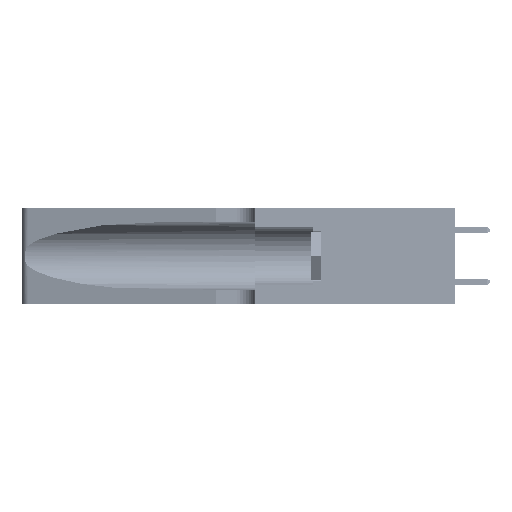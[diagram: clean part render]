
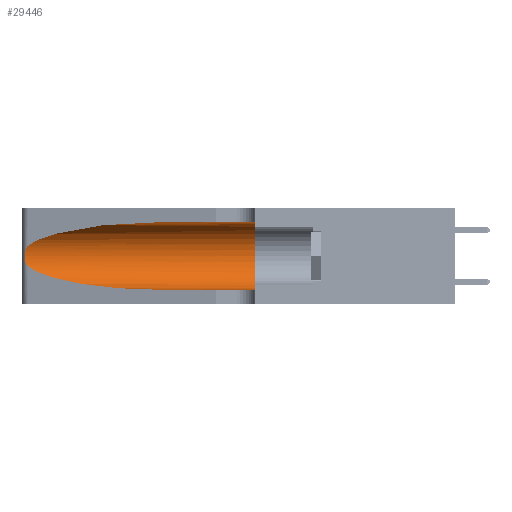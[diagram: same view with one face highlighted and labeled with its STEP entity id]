
A CAD part, left-side view. The second image highlights one B-rep face of the part: STEP entity #29446.
In plain terms, the highlighted cylindrical face has radius 3.308 mm (diameter 6.617 mm), a partial arc.
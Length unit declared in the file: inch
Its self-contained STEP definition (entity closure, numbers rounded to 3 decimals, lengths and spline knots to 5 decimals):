
#840 = ORIENTED_EDGE ( 'NONE', *, *, #49002, .T. ) ;
#1829 = DIRECTION ( 'NONE',  ( 0., 0., -1. ) ) ;
#2271 = EDGE_CURVE ( 'NONE', #34082, #46033, #19145, .T. ) ;
#2732 = LINE ( 'NONE', #43345, #43761 ) ;
#3081 = CARTESIAN_POINT ( 'NONE',  ( 0.25487, 1.22718, 0.22369 ) ) ;
#4306 = CARTESIAN_POINT ( 'NONE',  ( 0.25487, 1.22718, 0.14631 ) ) ;
#5226 = CARTESIAN_POINT ( 'NONE',  ( 0.1305, 0.35, 0.185 ) ) ;
#6212 = CARTESIAN_POINT ( 'NONE',  ( 0.1305, 0.72297, 0.31525 ) ) ;
#6383 = FACE_OUTER_BOUND ( 'NONE', #49997, .T. ) ;
#6954 = LINE ( 'NONE', #20405, #44265 ) ;
#7512 = CARTESIAN_POINT ( 'NONE',  ( 0.25856, 1.23593, 0.16098 ) ) ;
#7681 = CARTESIAN_POINT ( 'NONE',  ( 0.25487, 1.22718, 0.22369 ) ) ;
#7688 = CARTESIAN_POINT ( 'NONE',  ( 0.1305, 0.72297, 0.31525 ) ) ;
#9239 = DIRECTION ( 'NONE',  ( 0., 0., 1. ) ) ;
#9847 = ORIENTED_EDGE ( 'NONE', *, *, #13109, .F. ) ;
#11036 = CARTESIAN_POINT ( 'NONE',  ( 0.25639, 1.23186, 0.15144 ) ) ;
#11256 = ORIENTED_EDGE ( 'NONE', *, *, #45547, .T. ) ;
#13078 = VERTEX_POINT ( 'NONE', #16747 ) ;
#13109 = EDGE_CURVE ( 'NONE', #28854, #35072, #6954, .T. ) ;
#15540 = CARTESIAN_POINT ( 'NONE',  ( 0.25854, 1.2359, 0.20912 ) ) ;
#16747 = CARTESIAN_POINT ( 'NONE',  ( 0.1305, 0.35, 0.05475 ) ) ;
#17426 = CARTESIAN_POINT ( 'NONE',  ( 0.1305, 0.35, 0.31525 ) ) ;
#18692 = CIRCLE ( 'NONE', #24032, 0.13025 ) ;
#19145 = B_SPLINE_CURVE_WITH_KNOTS ( 'NONE', 3,
 ( #7681, #27005, #51390, #31512, #15540, #23680, #43154, #39186, #47032, #7512, #19354, #11036, #23522, #51221 ),
 .UNSPECIFIED., .F., .F.,
 ( 4, 2, 2, 2, 2, 2, 4 ),
 ( 0., 0.00027, 0.00053, 0.00107, 0.0016, 0.00187, 0.00214 ),
 .UNSPECIFIED. ) ;
#19354 = CARTESIAN_POINT ( 'NONE',  ( 0.25789, 1.23486, 0.15765 ) ) ;
#19531 = CARTESIAN_POINT ( 'NONE',  ( 0.2373, 1.15595, 0.28018 ) ) ;
#19809 = CARTESIAN_POINT ( 'NONE',  ( 0.18966, 0.96281, 0.05475 ) ) ;
#20405 = CARTESIAN_POINT ( 'NONE',  ( 0.1305, 1.61858, 0.31525 ) ) ;
#23061 = CARTESIAN_POINT ( 'NONE',  ( 0.25487, 1.22718, 0.14631 ) ) ;
#23522 = CARTESIAN_POINT ( 'NONE',  ( 0.25555, 1.22993, 0.14849 ) ) ;
#23680 = CARTESIAN_POINT ( 'NONE',  ( 0.26018, 1.23835, 0.19895 ) ) ;
#23696 = ORIENTED_EDGE ( 'NONE', *, *, #30982, .T. ) ;
#24032 = AXIS2_PLACEMENT_3D ( 'NONE', #5226, #36570, #9239 ) ;
#25633 = CARTESIAN_POINT ( 'NONE',  ( 0.1305, 1.61858, 0.185 ) ) ;
#27005 = CARTESIAN_POINT ( 'NONE',  ( 0.25555, 1.22994, 0.2215 ) ) ;
#28373 =( BOUNDED_CURVE ( )  B_SPLINE_CURVE ( 3, ( #7688, #47038, #19531, #43333 ),
 .UNSPECIFIED., .F., .F. ) 
 B_SPLINE_CURVE_WITH_KNOTS ( ( 4, 4 ),
 ( 1.5708, 2.84003 ),
 .UNSPECIFIED. ) 
 CURVE ( )  GEOMETRIC_REPRESENTATION_ITEM ( )  RATIONAL_B_SPLINE_CURVE ( ( 1., 0.87, 0.87, 1. ) ) 
 REPRESENTATION_ITEM ( '' )  );
#28854 = VERTEX_POINT ( 'NONE', #6212 ) ;
#29446 = ADVANCED_FACE ( 'NONE', ( #6383 ), #41865, .F. ) ;
#30982 = EDGE_CURVE ( 'NONE', #28854, #34082, #28373, .T. ) ;
#31512 = CARTESIAN_POINT ( 'NONE',  ( 0.25787, 1.23484, 0.2124 ) ) ;
#32303 = CARTESIAN_POINT ( 'NONE',  ( 0.2373, 1.15595, 0.08982 ) ) ;
#33391 = ORIENTED_EDGE ( 'NONE', *, *, #43153, .F. ) ;
#34082 = VERTEX_POINT ( 'NONE', #3081 ) ;
#35072 = VERTEX_POINT ( 'NONE', #17426 ) ;
#36570 = DIRECTION ( 'NONE',  ( 0., 1., 0. ) ) ;
#38183 = CARTESIAN_POINT ( 'NONE',  ( 0.1305, 0.72297, 0.05475 ) ) ;
#39186 = CARTESIAN_POINT ( 'NONE',  ( 0.26075, 1.23896, 0.178 ) ) ;
#39803 = CARTESIAN_POINT ( 'NONE',  ( 0.1305, 0.72297, 0.05475 ) ) ;
#40378 = DIRECTION ( 'NONE',  ( 0., -1., 0. ) ) ;
#41865 = CYLINDRICAL_SURFACE ( 'NONE', #49493, 0.13025 ) ;
#42395 =( BOUNDED_CURVE ( )  B_SPLINE_CURVE ( 3, ( #4306, #32303, #19809, #39803 ),
 .UNSPECIFIED., .F., .T. ) 
 B_SPLINE_CURVE_WITH_KNOTS ( ( 4, 4 ),
 ( 3.44316, 4.71239 ),
 .UNSPECIFIED. ) 
 CURVE ( )  GEOMETRIC_REPRESENTATION_ITEM ( )  RATIONAL_B_SPLINE_CURVE ( ( 1., 0.87, 0.87, 1. ) ) 
 REPRESENTATION_ITEM ( '' )  );
#43153 = EDGE_CURVE ( 'NONE', #35072, #13078, #18692, .T. ) ;
#43154 = CARTESIAN_POINT ( 'NONE',  ( 0.26075, 1.23896, 0.19203 ) ) ;
#43333 = CARTESIAN_POINT ( 'NONE',  ( 0.25487, 1.22718, 0.22369 ) ) ;
#43345 = CARTESIAN_POINT ( 'NONE',  ( 0.1305, 1.61858, 0.05475 ) ) ;
#43507 = DIRECTION ( 'NONE',  ( 0., -1., 0. ) ) ;
#43761 = VECTOR ( 'NONE', #43507, 39.37008 ) ;
#44265 = VECTOR ( 'NONE', #40378, 39.37008 ) ;
#45547 = EDGE_CURVE ( 'NONE', #46033, #46734, #42395, .T. ) ;
#46033 = VERTEX_POINT ( 'NONE', #23061 ) ;
#46734 = VERTEX_POINT ( 'NONE', #38183 ) ;
#47032 = CARTESIAN_POINT ( 'NONE',  ( 0.26017, 1.23833, 0.17102 ) ) ;
#47038 = CARTESIAN_POINT ( 'NONE',  ( 0.18966, 0.96281, 0.31525 ) ) ;
#48053 = ORIENTED_EDGE ( 'NONE', *, *, #2271, .T. ) ;
#49002 = EDGE_CURVE ( 'NONE', #46734, #13078, #2732, .T. ) ;
#49493 = AXIS2_PLACEMENT_3D ( 'NONE', #25633, #50010, #1829 ) ;
#49997 = EDGE_LOOP ( 'NONE', ( #23696, #48053, #11256, #840, #33391, #9847 ) ) ;
#50010 = DIRECTION ( 'NONE',  ( 0., -1., 0. ) ) ;
#51221 = CARTESIAN_POINT ( 'NONE',  ( 0.25487, 1.22718, 0.14631 ) ) ;
#51390 = CARTESIAN_POINT ( 'NONE',  ( 0.25639, 1.23184, 0.21858 ) ) ;
